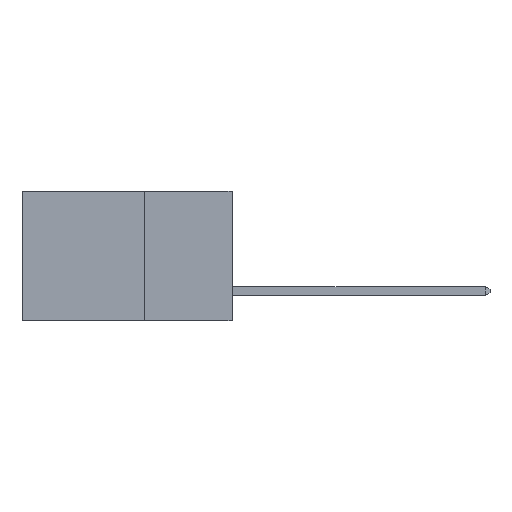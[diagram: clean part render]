
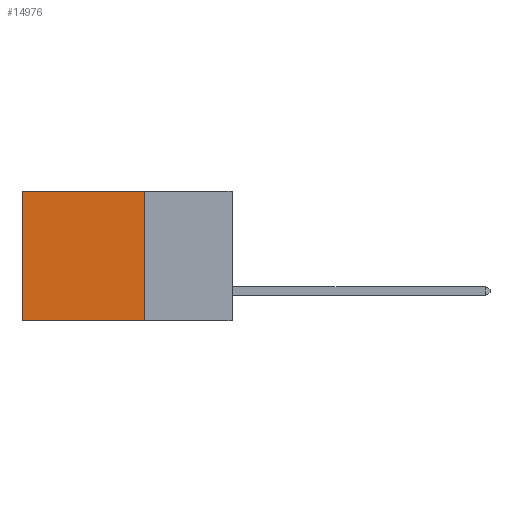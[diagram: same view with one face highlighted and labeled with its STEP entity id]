
A CAD part, left-side view. The second image highlights one B-rep face of the part: STEP entity #14976.
In plain terms, the highlighted planar face has unit normal (-1, 0, 0).
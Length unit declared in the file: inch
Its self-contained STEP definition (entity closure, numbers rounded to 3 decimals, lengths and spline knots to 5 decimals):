
#592 = VERTEX_POINT ( 'NONE', #1860 ) ;
#954 = CARTESIAN_POINT ( 'NONE',  ( 0.2875, 0.25, 0. ) ) ;
#1860 = CARTESIAN_POINT ( 'NONE',  ( 0.2875, 0.25, 0. ) ) ;
#1890 = LINE ( 'NONE', #18594, #17780 ) ;
#2131 = CARTESIAN_POINT ( 'NONE',  ( 0.2875, 0.25, 0. ) ) ;
#3010 = DIRECTION ( 'NONE',  ( 1., 0., 0. ) ) ;
#4058 = EDGE_LOOP ( 'NONE', ( #13044, #20921, #5463, #10038 ) ) ;
#5463 = ORIENTED_EDGE ( 'NONE', *, *, #24993, .F. ) ;
#6149 = DIRECTION ( 'NONE',  ( 0., 0., -1. ) ) ;
#8191 = CARTESIAN_POINT ( 'NONE',  ( 0.2875, 0.6, 0. ) ) ;
#10038 = ORIENTED_EDGE ( 'NONE', *, *, #22755, .T. ) ;
#11691 = LINE ( 'NONE', #8191, #12304 ) ;
#12304 = VECTOR ( 'NONE', #22106, 39.37008 ) ;
#12836 = PLANE ( 'NONE',  #22808 ) ;
#13044 = ORIENTED_EDGE ( 'NONE', *, *, #17382, .T. ) ;
#13338 = DIRECTION ( 'NONE',  ( 0., 1., 0. ) ) ;
#14135 = CARTESIAN_POINT ( 'NONE',  ( 0.2875, 0.6, -0.37 ) ) ;
#14976 = ADVANCED_FACE ( 'NONE', ( #17504 ), #12836, .F. ) ;
#16481 = EDGE_CURVE ( 'NONE', #23639, #25301, #22364, .T. ) ;
#16896 = DIRECTION ( 'NONE',  ( 0., 0., -1. ) ) ;
#17102 = VECTOR ( 'NONE', #13338, 39.37008 ) ;
#17382 = EDGE_CURVE ( 'NONE', #25188, #25301, #11691, .T. ) ;
#17504 = FACE_OUTER_BOUND ( 'NONE', #4058, .T. ) ;
#17780 = VECTOR ( 'NONE', #22678, 39.37008 ) ;
#18594 = CARTESIAN_POINT ( 'NONE',  ( 0.2875, 0.25, 0. ) ) ;
#18648 = CARTESIAN_POINT ( 'NONE',  ( 0.2875, 0.6, 0. ) ) ;
#19282 = CARTESIAN_POINT ( 'NONE',  ( 0.2875, 0.25, -0.37 ) ) ;
#20079 = VECTOR ( 'NONE', #6149, 39.37008 ) ;
#20715 = LINE ( 'NONE', #2131, #20079 ) ;
#20921 = ORIENTED_EDGE ( 'NONE', *, *, #16481, .F. ) ;
#22106 = DIRECTION ( 'NONE',  ( 0., 0., -1. ) ) ;
#22364 = LINE ( 'NONE', #19282, #17102 ) ;
#22678 = DIRECTION ( 'NONE',  ( 0., 1., 0. ) ) ;
#22755 = EDGE_CURVE ( 'NONE', #592, #25188, #1890, .T. ) ;
#22808 = AXIS2_PLACEMENT_3D ( 'NONE', #954, #3010, #16896 ) ;
#23639 = VERTEX_POINT ( 'NONE', #25479 ) ;
#24993 = EDGE_CURVE ( 'NONE', #592, #23639, #20715, .T. ) ;
#25188 = VERTEX_POINT ( 'NONE', #18648 ) ;
#25301 = VERTEX_POINT ( 'NONE', #14135 ) ;
#25479 = CARTESIAN_POINT ( 'NONE',  ( 0.2875, 0.25, -0.37 ) ) ;
